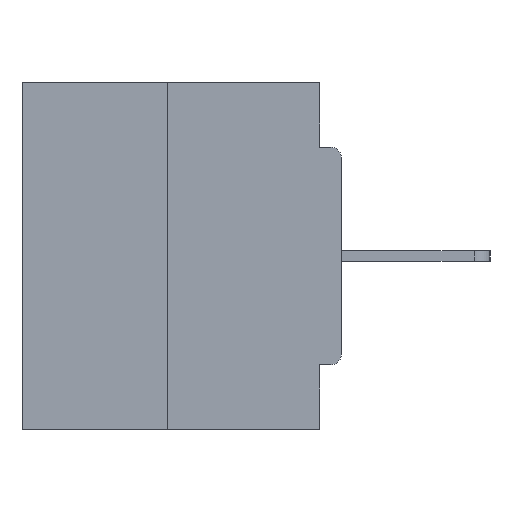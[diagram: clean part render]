
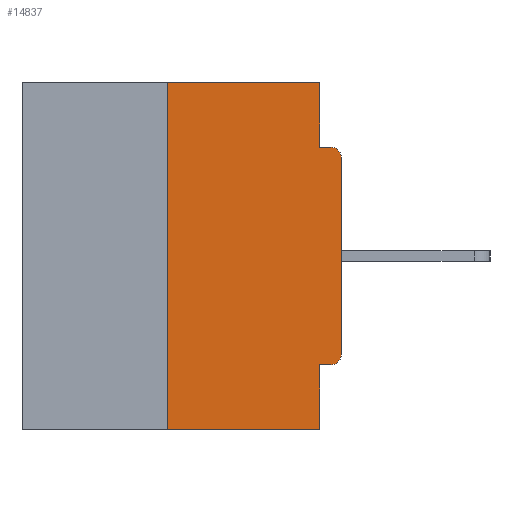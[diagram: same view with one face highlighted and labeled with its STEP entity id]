
A CAD part, left-side view. The second image highlights one B-rep face of the part: STEP entity #14837.
In plain terms, the highlighted planar face has unit normal (-1, 0, 0).
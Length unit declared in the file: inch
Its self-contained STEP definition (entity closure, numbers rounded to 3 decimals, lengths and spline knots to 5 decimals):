
#814 = CARTESIAN_POINT ( 'NONE',  ( 0., 0.031, -0.0935 ) ) ;
#1031 = CARTESIAN_POINT ( 'NONE',  ( 0., 0.46, -0.5 ) ) ;
#1121 = VERTEX_POINT ( 'NONE', #29482 ) ;
#1774 = VERTEX_POINT ( 'NONE', #2612 ) ;
#1828 = CARTESIAN_POINT ( 'NONE',  ( 0., 0.015, -0.3915 ) ) ;
#2516 = CARTESIAN_POINT ( 'NONE',  ( 0., 0., 0. ) ) ;
#2612 = CARTESIAN_POINT ( 'NONE',  ( 0., 0.015, -0.4065 ) ) ;
#3310 = DIRECTION ( 'NONE',  ( 0., -1., 0. ) ) ;
#3645 = VERTEX_POINT ( 'NONE', #32264 ) ;
#4368 = DIRECTION ( 'NONE',  ( 0., -1., 0. ) ) ;
#4397 = EDGE_LOOP ( 'NONE', ( #5700, #14130, #6355, #14025, #11826, #13760, #12565, #21480, #6289, #7428 ) ) ;
#4436 = DIRECTION ( 'NONE',  ( 0., 0., -1. ) ) ;
#4783 = CARTESIAN_POINT ( 'NONE',  ( 0., 0.031, 0. ) ) ;
#4853 = CARTESIAN_POINT ( 'NONE',  ( 0., 0., -0.1085 ) ) ;
#5700 = ORIENTED_EDGE ( 'NONE', *, *, #7737, .F. ) ;
#5827 = VECTOR ( 'NONE', #3310, 39.37008 ) ;
#5902 = CARTESIAN_POINT ( 'NONE',  ( 0., 0.46, 0. ) ) ;
#6139 = CARTESIAN_POINT ( 'NONE',  ( 0., 0.25, 0. ) ) ;
#6289 = ORIENTED_EDGE ( 'NONE', *, *, #23647, .F. ) ;
#6355 = ORIENTED_EDGE ( 'NONE', *, *, #29793, .T. ) ;
#6590 = LINE ( 'NONE', #30126, #10349 ) ;
#6592 = EDGE_CURVE ( 'NONE', #3645, #15212, #30874, .T. ) ;
#7084 = LINE ( 'NONE', #17046, #14808 ) ;
#7428 = ORIENTED_EDGE ( 'NONE', *, *, #6592, .F. ) ;
#7737 = EDGE_CURVE ( 'NONE', #31186, #3645, #14100, .T. ) ;
#7827 = LINE ( 'NONE', #2516, #17071 ) ;
#9539 = VECTOR ( 'NONE', #4436, 39.37008 ) ;
#9713 = VERTEX_POINT ( 'NONE', #15292 ) ;
#10349 = VECTOR ( 'NONE', #22229, 39.37008 ) ;
#11091 = AXIS2_PLACEMENT_3D ( 'NONE', #22991, #22825, #18167 ) ;
#11462 = FACE_OUTER_BOUND ( 'NONE', #4397, .T. ) ;
#11475 = DIRECTION ( 'NONE',  ( 0., -1., 0. ) ) ;
#11596 = DIRECTION ( 'NONE',  ( 0., 0., 1. ) ) ;
#11826 = ORIENTED_EDGE ( 'NONE', *, *, #28880, .F. ) ;
#12214 = DIRECTION ( 'NONE',  ( 0., 1., 0. ) ) ;
#12314 = CARTESIAN_POINT ( 'NONE',  ( 0., 0.25, 0. ) ) ;
#12565 = ORIENTED_EDGE ( 'NONE', *, *, #30363, .T. ) ;
#12788 = EDGE_CURVE ( 'NONE', #1774, #19963, #21881, .T. ) ;
#13760 = ORIENTED_EDGE ( 'NONE', *, *, #12788, .T. ) ;
#14025 = ORIENTED_EDGE ( 'NONE', *, *, #23479, .F. ) ;
#14100 = LINE ( 'NONE', #5902, #5827 ) ;
#14130 = ORIENTED_EDGE ( 'NONE', *, *, #27518, .F. ) ;
#14223 = CARTESIAN_POINT ( 'NONE',  ( 0., 0., -0.3915 ) ) ;
#14808 = VECTOR ( 'NONE', #12214, 39.37008 ) ;
#14837 = ADVANCED_FACE ( 'NONE', ( #11462 ), #21956, .F. ) ;
#15212 = VERTEX_POINT ( 'NONE', #814 ) ;
#15292 = CARTESIAN_POINT ( 'NONE',  ( 0., 0.25, -0.5 ) ) ;
#16229 = DIRECTION ( 'NONE',  ( 0., 0., 1. ) ) ;
#16534 = AXIS2_PLACEMENT_3D ( 'NONE', #26791, #19367, #24045 ) ;
#17046 = CARTESIAN_POINT ( 'NONE',  ( 0., 0., -0.4065 ) ) ;
#17071 = VECTOR ( 'NONE', #16229, 39.37008 ) ;
#18167 = DIRECTION ( 'NONE',  ( 0., 0., -1. ) ) ;
#19043 = CARTESIAN_POINT ( 'NONE',  ( 0., 0.015, -0.0935 ) ) ;
#19214 = LINE ( 'NONE', #1031, #25839 ) ;
#19367 = DIRECTION ( 'NONE',  ( 1., 0., 0. ) ) ;
#19963 = VERTEX_POINT ( 'NONE', #14223 ) ;
#20370 = DIRECTION ( 'NONE',  ( 0., 0., -1. ) ) ;
#20608 = VERTEX_POINT ( 'NONE', #26693 ) ;
#20972 = CARTESIAN_POINT ( 'NONE',  ( 0., 0., -0.0935 ) ) ;
#21480 = ORIENTED_EDGE ( 'NONE', *, *, #31213, .T. ) ;
#21881 = CIRCLE ( 'NONE', #25732, 0.015 ) ;
#21956 = PLANE ( 'NONE',  #16534 ) ;
#22229 = DIRECTION ( 'NONE',  ( 0., 0., -1. ) ) ;
#22825 = DIRECTION ( 'NONE',  ( -1., 0., 0. ) ) ;
#22991 = CARTESIAN_POINT ( 'NONE',  ( 0., 0.015, -0.1085 ) ) ;
#23479 = EDGE_CURVE ( 'NONE', #1121, #20608, #6590, .T. ) ;
#23647 = EDGE_CURVE ( 'NONE', #15212, #32471, #28061, .T. ) ;
#24045 = DIRECTION ( 'NONE',  ( 0., 0., -1. ) ) ;
#24165 = VECTOR ( 'NONE', #11596, 39.37008 ) ;
#25732 = AXIS2_PLACEMENT_3D ( 'NONE', #1828, #33577, #20370 ) ;
#25839 = VECTOR ( 'NONE', #11475, 39.37008 ) ;
#26693 = CARTESIAN_POINT ( 'NONE',  ( 0., 0.031, -0.5 ) ) ;
#26791 = CARTESIAN_POINT ( 'NONE',  ( 0., 0.46, 0. ) ) ;
#27250 = LINE ( 'NONE', #6139, #24165 ) ;
#27518 = EDGE_CURVE ( 'NONE', #9713, #31186, #27250, .T. ) ;
#28061 = LINE ( 'NONE', #20972, #30649 ) ;
#28880 = EDGE_CURVE ( 'NONE', #1774, #1121, #7084, .T. ) ;
#29482 = CARTESIAN_POINT ( 'NONE',  ( 0., 0.031, -0.4065 ) ) ;
#29793 = EDGE_CURVE ( 'NONE', #9713, #20608, #19214, .T. ) ;
#30126 = CARTESIAN_POINT ( 'NONE',  ( 0., 0.031, -0.5 ) ) ;
#30363 = EDGE_CURVE ( 'NONE', #19963, #32629, #7827, .T. ) ;
#30649 = VECTOR ( 'NONE', #4368, 39.37008 ) ;
#30874 = LINE ( 'NONE', #4783, #9539 ) ;
#31186 = VERTEX_POINT ( 'NONE', #12314 ) ;
#31213 = EDGE_CURVE ( 'NONE', #32629, #32471, #31411, .T. ) ;
#31411 = CIRCLE ( 'NONE', #11091, 0.015 ) ;
#32264 = CARTESIAN_POINT ( 'NONE',  ( 0., 0.031, 0. ) ) ;
#32471 = VERTEX_POINT ( 'NONE', #19043 ) ;
#32629 = VERTEX_POINT ( 'NONE', #4853 ) ;
#33577 = DIRECTION ( 'NONE',  ( -1., 0., 0. ) ) ;
